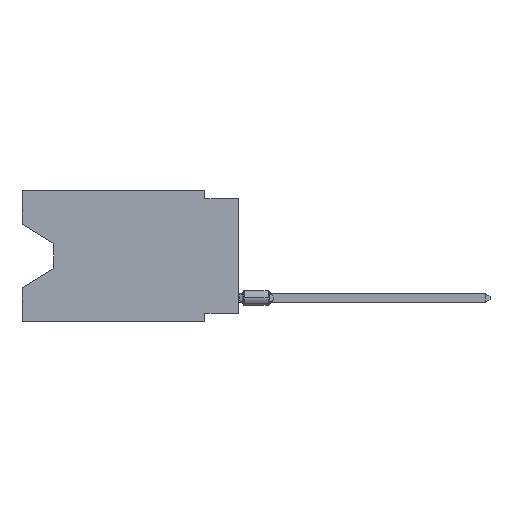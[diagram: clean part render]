
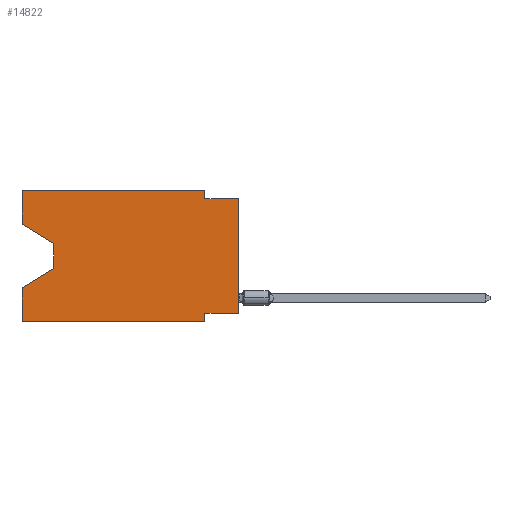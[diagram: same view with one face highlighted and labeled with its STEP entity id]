
A CAD part, left-side view. The second image highlights one B-rep face of the part: STEP entity #14822.
In plain terms, the highlighted planar face has unit normal (-1, 0, 0).
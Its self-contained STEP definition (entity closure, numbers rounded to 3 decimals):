
#33 = VERTEX_POINT ( 'NONE', #6777 ) ;
#70 = DIRECTION ( 'NONE',  ( 0., 0., 1. ) ) ;
#483 = DIRECTION ( 'NONE',  ( 0., 0.855, -0.519 ) ) ;
#1000 = EDGE_CURVE ( 'NONE', #11890, #20868, #23587, .T. ) ;
#1083 = EDGE_CURVE ( 'NONE', #11083, #29577, #14564, .T. ) ;
#1670 = CARTESIAN_POINT ( 'NONE',  ( 0., 0., -0.635 ) ) ;
#1706 = CARTESIAN_POINT ( 'NONE',  ( 0., 16.383, 0. ) ) ;
#2138 = EDGE_LOOP ( 'NONE', ( #18164, #18122, #21561, #17628, #25419, #16233, #17275, #27497, #13747, #19765, #11428, #19427 ) ) ;
#2955 = DIRECTION ( 'NONE',  ( 0., 0., -1. ) ) ;
#3052 = VECTOR ( 'NONE', #483, 1000. ) ;
#4171 = VERTEX_POINT ( 'NONE', #18877 ) ;
#4479 = EDGE_CURVE ( 'NONE', #4171, #18052, #28437, .T. ) ;
#4508 = VECTOR ( 'NONE', #14957, 1000. ) ;
#4585 = CARTESIAN_POINT ( 'NONE',  ( 0., 16.383, -7.36 ) ) ;
#4709 = LINE ( 'NONE', #28102, #26629 ) ;
#5481 = CARTESIAN_POINT ( 'NONE',  ( 0., 13.97, -4.013 ) ) ;
#5513 = LINE ( 'NONE', #12327, #4508 ) ;
#6642 = CARTESIAN_POINT ( 'NONE',  ( 0., 2.54, -9.271 ) ) ;
#6762 = LINE ( 'NONE', #11103, #15368 ) ;
#6777 = CARTESIAN_POINT ( 'NONE',  ( 0., 2.54, 0. ) ) ;
#7224 = CARTESIAN_POINT ( 'NONE',  ( 0., 16.383, -9.906 ) ) ;
#7450 = DIRECTION ( 'NONE',  ( 0., 0., -1. ) ) ;
#7618 = LINE ( 'NONE', #9925, #3052 ) ;
#8482 = DIRECTION ( 'NONE',  ( 0., 0., -1. ) ) ;
#9772 = CARTESIAN_POINT ( 'NONE',  ( 0., 16.383, 0. ) ) ;
#9859 = VERTEX_POINT ( 'NONE', #11789 ) ;
#9925 = CARTESIAN_POINT ( 'NONE',  ( 0., 13.97, -5.893 ) ) ;
#10322 = VECTOR ( 'NONE', #23653, 1000. ) ;
#10890 = LINE ( 'NONE', #22515, #28808 ) ;
#11083 = VERTEX_POINT ( 'NONE', #5481 ) ;
#11103 = CARTESIAN_POINT ( 'NONE',  ( 0., 2.54, 0. ) ) ;
#11424 = CARTESIAN_POINT ( 'NONE',  ( 0., 0., -0.635 ) ) ;
#11428 = ORIENTED_EDGE ( 'NONE', *, *, #30636, .F. ) ;
#11789 = CARTESIAN_POINT ( 'NONE',  ( 0., 16.383, -9.906 ) ) ;
#11890 = VERTEX_POINT ( 'NONE', #13708 ) ;
#12066 = VECTOR ( 'NONE', #16617, 1000. ) ;
#12327 = CARTESIAN_POINT ( 'NONE',  ( 0., 16.383, 0. ) ) ;
#12348 = EDGE_CURVE ( 'NONE', #23819, #14220, #18560, .T. ) ;
#12752 = AXIS2_PLACEMENT_3D ( 'NONE', #17054, #26500, #2955 ) ;
#13514 = VECTOR ( 'NONE', #18843, 1000. ) ;
#13708 = CARTESIAN_POINT ( 'NONE',  ( 0., 16.383, -2.546 ) ) ;
#13747 = ORIENTED_EDGE ( 'NONE', *, *, #12348, .F. ) ;
#14220 = VERTEX_POINT ( 'NONE', #1670 ) ;
#14564 = LINE ( 'NONE', #28677, #24712 ) ;
#14822 = ADVANCED_FACE ( 'NONE', ( #21856 ), #23743, .F. ) ;
#14957 = DIRECTION ( 'NONE',  ( 0., -1., 0. ) ) ;
#15036 = DIRECTION ( 'NONE',  ( 0., -0.855, -0.519 ) ) ;
#15368 = VECTOR ( 'NONE', #8482, 1000. ) ;
#16233 = ORIENTED_EDGE ( 'NONE', *, *, #20509, .F. ) ;
#16469 = LINE ( 'NONE', #19108, #12066 ) ;
#16617 = DIRECTION ( 'NONE',  ( 0., 0., 1. ) ) ;
#17054 = CARTESIAN_POINT ( 'NONE',  ( 0., 16.383, 0. ) ) ;
#17275 = ORIENTED_EDGE ( 'NONE', *, *, #4479, .F. ) ;
#17628 = ORIENTED_EDGE ( 'NONE', *, *, #27186, .F. ) ;
#18052 = VERTEX_POINT ( 'NONE', #6642 ) ;
#18122 = ORIENTED_EDGE ( 'NONE', *, *, #1083, .T. ) ;
#18124 = CARTESIAN_POINT ( 'NONE',  ( 0., 2.54, -9.906 ) ) ;
#18164 = ORIENTED_EDGE ( 'NONE', *, *, #30149, .T. ) ;
#18541 = CARTESIAN_POINT ( 'NONE',  ( 0., 0., -9.271 ) ) ;
#18560 = LINE ( 'NONE', #11424, #24015 ) ;
#18843 = DIRECTION ( 'NONE',  ( 0., -1., 0. ) ) ;
#18877 = CARTESIAN_POINT ( 'NONE',  ( 0., 0., -9.271 ) ) ;
#19108 = CARTESIAN_POINT ( 'NONE',  ( 0., 16.383, 0. ) ) ;
#19427 = ORIENTED_EDGE ( 'NONE', *, *, #1000, .F. ) ;
#19530 = EDGE_CURVE ( 'NONE', #33, #23819, #6762, .T. ) ;
#19701 = LINE ( 'NONE', #21697, #23014 ) ;
#19765 = ORIENTED_EDGE ( 'NONE', *, *, #19530, .F. ) ;
#20509 = EDGE_CURVE ( 'NONE', #18052, #22485, #10890, .T. ) ;
#20779 = EDGE_CURVE ( 'NONE', #29577, #24880, #7618, .T. ) ;
#20868 = VERTEX_POINT ( 'NONE', #1706 ) ;
#21242 = DIRECTION ( 'NONE',  ( 0., 0., 1. ) ) ;
#21324 = DIRECTION ( 'NONE',  ( 0., -1., 0. ) ) ;
#21561 = ORIENTED_EDGE ( 'NONE', *, *, #20779, .T. ) ;
#21697 = CARTESIAN_POINT ( 'NONE',  ( 0., 16.383, -2.546 ) ) ;
#21727 = EDGE_CURVE ( 'NONE', #9859, #22485, #23958, .T. ) ;
#21856 = FACE_OUTER_BOUND ( 'NONE', #2138, .T. ) ;
#22485 = VERTEX_POINT ( 'NONE', #18124 ) ;
#22515 = CARTESIAN_POINT ( 'NONE',  ( 0., 2.54, -9.906 ) ) ;
#23014 = VECTOR ( 'NONE', #15036, 1000. ) ;
#23587 = LINE ( 'NONE', #9772, #25192 ) ;
#23653 = DIRECTION ( 'NONE',  ( 0., 1., 0. ) ) ;
#23743 = PLANE ( 'NONE',  #12752 ) ;
#23819 = VERTEX_POINT ( 'NONE', #27014 ) ;
#23958 = LINE ( 'NONE', #7224, #13514 ) ;
#24015 = VECTOR ( 'NONE', #21324, 1000. ) ;
#24712 = VECTOR ( 'NONE', #7450, 1000. ) ;
#24880 = VERTEX_POINT ( 'NONE', #4585 ) ;
#25192 = VECTOR ( 'NONE', #21242, 1000. ) ;
#25368 = EDGE_CURVE ( 'NONE', #4171, #14220, #4709, .T. ) ;
#25419 = ORIENTED_EDGE ( 'NONE', *, *, #21727, .T. ) ;
#25946 = CARTESIAN_POINT ( 'NONE',  ( 0., 13.97, -5.893 ) ) ;
#26500 = DIRECTION ( 'NONE',  ( 1., 0., 0. ) ) ;
#26629 = VECTOR ( 'NONE', #70, 1000. ) ;
#27014 = CARTESIAN_POINT ( 'NONE',  ( 0., 2.54, -0.635 ) ) ;
#27186 = EDGE_CURVE ( 'NONE', #9859, #24880, #16469, .T. ) ;
#27497 = ORIENTED_EDGE ( 'NONE', *, *, #25368, .T. ) ;
#28102 = CARTESIAN_POINT ( 'NONE',  ( 0., 0., 0. ) ) ;
#28437 = LINE ( 'NONE', #18541, #10322 ) ;
#28677 = CARTESIAN_POINT ( 'NONE',  ( 0., 13.97, -4.013 ) ) ;
#28808 = VECTOR ( 'NONE', #29790, 1000. ) ;
#29577 = VERTEX_POINT ( 'NONE', #25946 ) ;
#29790 = DIRECTION ( 'NONE',  ( 0., 0., -1. ) ) ;
#30149 = EDGE_CURVE ( 'NONE', #11890, #11083, #19701, .T. ) ;
#30636 = EDGE_CURVE ( 'NONE', #20868, #33, #5513, .T. ) ;
